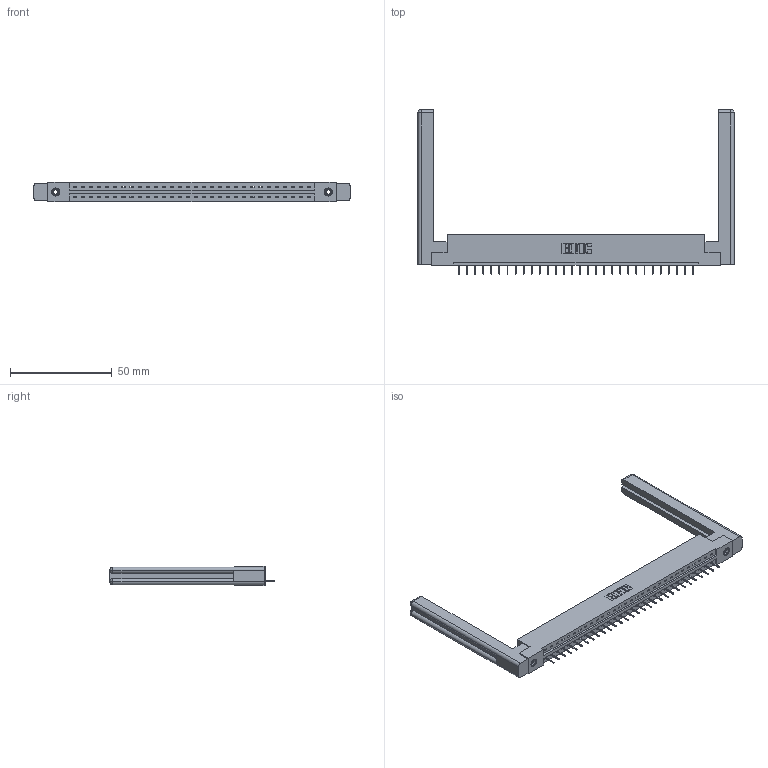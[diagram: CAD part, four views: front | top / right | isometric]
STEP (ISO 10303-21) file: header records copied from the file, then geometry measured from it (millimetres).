
FILE_DESCRIPTION (( 'STEP AP203' ), '1' );
FILE_NAME ('387-030-524-158.STEP', '2019-10-03T18:04:35', ( '' ), ( '' ), 'SwSTEP 2.0', 'SolidWorks 2016', '' );
FILE_SCHEMA (( 'CONFIG_CONTROL_DESIGN' ));
Length unit declared in the file: inch
Products named in the file (5): 345-292-001_345-293-124; 337 Part_Flush Mounting Lugs - 0.156 Dia-TI; 345-250-001_345-250-001-102; 387-030-524-158; 307-220-058
Assembly tree (35 placements, depth 2):
  387-030-524-158
    337 Part_Flush Mounting Lugs - 0.156 Dia-TI
    345-292-001_345-293-124  x30
    345-250-001_345-250-001-102  x2
    307-220-058  x2
Bounding box: 155.5 x 80.78 x 9.4 mm (x, y, z)
Volume: 23055 mm3; surface area: 21152.6 mm2
Topology: 35 solids, 35 shells, 2236 faces, 6425 edges, 4150 vertices
Faces by surface type: plane 1714, cylinder 498, cone 12, torus 12
Entity records: 26560 total; most frequent: CARTESIAN_POINT 4623, ORIENTED_EDGE 4528, DIRECTION 3936, EDGE_CURVE 2264, VECTOR 2092, LINE 2092, VERTEX_POINT 1498, AXIS2_PLACEMENT_3D 922
